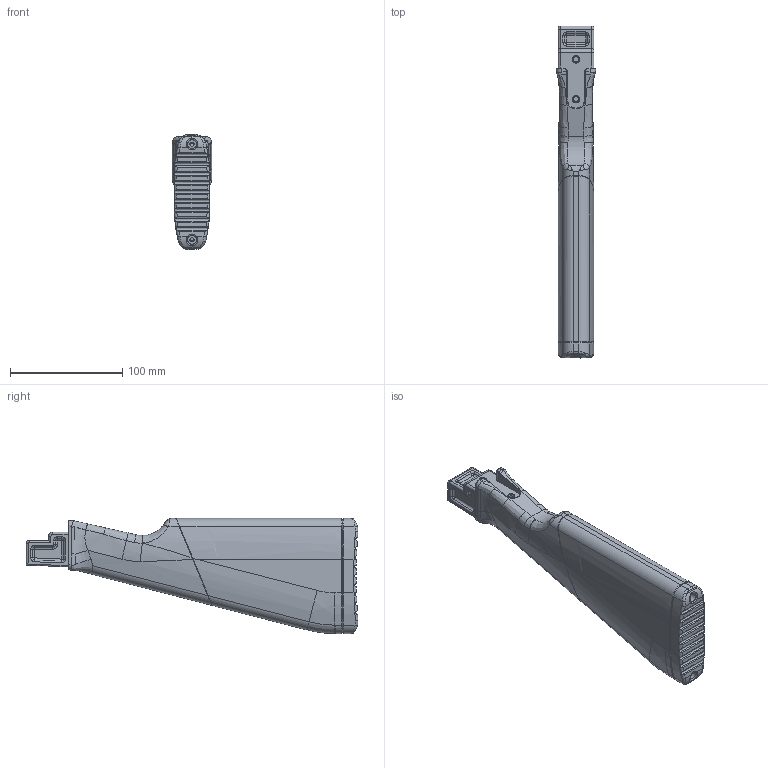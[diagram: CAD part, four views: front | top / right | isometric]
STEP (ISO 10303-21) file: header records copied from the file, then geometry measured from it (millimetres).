
FILE_DESCRIPTION(/* description */ (''),/* implementation_level */ '2;1');
FILE_NAME(/* name */ 'Spilt Stock.step',/* time_stamp */ '2021-09-27T04:30:49-04:00',/* author */ (''),/* organization */ (''),/* preprocessor_version */ 'ST-DEVELOPER v18.1',/* originating_system */ 'Autodesk Translation Framework v10.10.0.1391',/* authorisation */ '');
FILE_SCHEMA (('AUTOMOTIVE_DESIGN { 1 0 10303 214 3 1 1 }'));
Length unit declared in the file: millimetre
Products named in the file (1): Spilt Stock
Bounding box: 35 x 295.71 x 102.57 mm (x, y, z)
Volume: 336879.7 mm3; surface area: 101426 mm2
Topology: 3 solids, 5 shells, 715 faces, 1722 edges, 1026 vertices
Faces by surface type: bspline 246, cylinder 233, plane 99, torus 75, cone 40, sphere 22
Full cylindrical faces by diameter (mm): 3.7 x4, 4.6 x2, 6.7 x14, 8 x2
Entity records: 57882 total; most frequent: CARTESIAN_POINT 42693, ORIENTED_EDGE 3414, DIRECTION 2752, EDGE_CURVE 1707, AXIS2_PLACEMENT_3D 1136, VERTEX_POINT 1026, EDGE_LOOP 749, FACE_OUTER_BOUND 715
